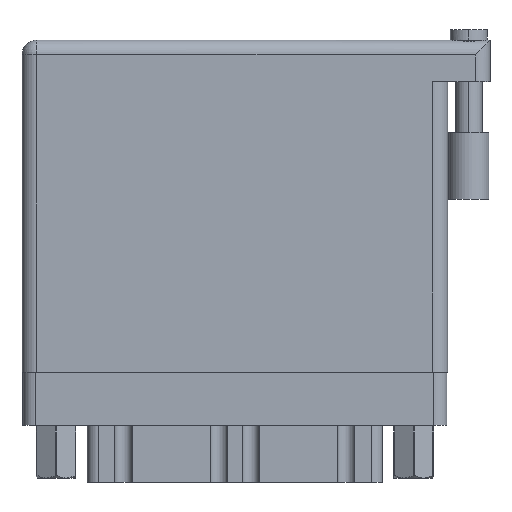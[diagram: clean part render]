
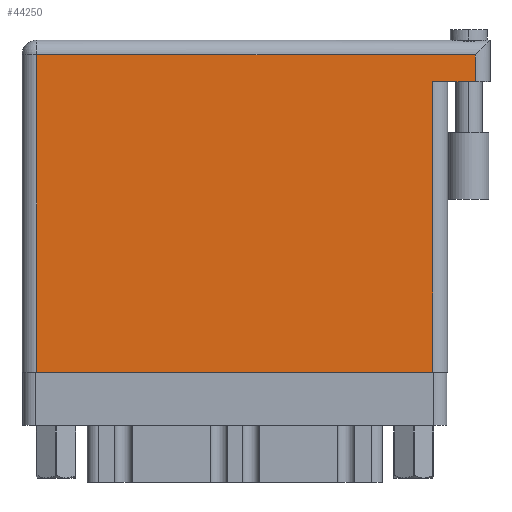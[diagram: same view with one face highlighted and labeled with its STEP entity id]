
A CAD part, front view. The second image highlights one B-rep face of the part: STEP entity #44250.
In plain terms, the highlighted face is planar.
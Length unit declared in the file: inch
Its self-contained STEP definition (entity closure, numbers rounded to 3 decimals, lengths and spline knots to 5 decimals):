
#753 = LINE ( 'NONE', #29842, #9452 ) ;
#2338 = VERTEX_POINT ( 'NONE', #11814 ) ;
#2856 = DIRECTION ( 'NONE',  ( 0., 1., 0. ) ) ;
#3037 = CARTESIAN_POINT ( 'NONE',  ( 0.07, 0., 0. ) ) ;
#3648 = CARTESIAN_POINT ( 'NONE',  ( 2.138, 1.496, 0. ) ) ;
#4617 = VECTOR ( 'NONE', #2856, 39.37008 ) ;
#7962 = VECTOR ( 'NONE', #34543, 39.37008 ) ;
#8589 = CARTESIAN_POINT ( 'NONE',  ( 0.07, 0., 0. ) ) ;
#8846 = VERTEX_POINT ( 'NONE', #3648 ) ;
#9449 = CARTESIAN_POINT ( 'NONE',  ( 0., 1.566, 0. ) ) ;
#9452 = VECTOR ( 'NONE', #19588, 39.37008 ) ;
#10543 = ORIENTED_EDGE ( 'NONE', *, *, #22997, .T. ) ;
#10913 = VERTEX_POINT ( 'NONE', #41477 ) ;
#10958 = CARTESIAN_POINT ( 'NONE',  ( 2.138, 1.566, 0. ) ) ;
#11483 = CARTESIAN_POINT ( 'NONE',  ( 1.938, 0., 0. ) ) ;
#11814 = CARTESIAN_POINT ( 'NONE',  ( 1.938, 1.369, 0. ) ) ;
#13373 = VECTOR ( 'NONE', #24714, 39.37008 ) ;
#13679 = EDGE_CURVE ( 'NONE', #39308, #15111, #753, .T. ) ;
#15111 = VERTEX_POINT ( 'NONE', #11483 ) ;
#15180 = LINE ( 'NONE', #41134, #33254 ) ;
#16439 = LINE ( 'NONE', #35491, #7962 ) ;
#16831 = DIRECTION ( 'NONE',  ( 0., 0., -1. ) ) ;
#17113 = EDGE_CURVE ( 'NONE', #8846, #10913, #31848, .T. ) ;
#19588 = DIRECTION ( 'NONE',  ( 1., 0., 0. ) ) ;
#20398 = DIRECTION ( 'NONE',  ( -1., 0., 0. ) ) ;
#22274 = ORIENTED_EDGE ( 'NONE', *, *, #25576, .T. ) ;
#22997 = EDGE_CURVE ( 'NONE', #26460, #8846, #24798, .T. ) ;
#24198 = ORIENTED_EDGE ( 'NONE', *, *, #46103, .F. ) ;
#24227 = PLANE ( 'NONE',  #34693 ) ;
#24714 = DIRECTION ( 'NONE',  ( -1., 0., 0. ) ) ;
#24798 = LINE ( 'NONE', #10958, #4617 ) ;
#25576 = EDGE_CURVE ( 'NONE', #15111, #2338, #16439, .T. ) ;
#26460 = VERTEX_POINT ( 'NONE', #27039 ) ;
#27039 = CARTESIAN_POINT ( 'NONE',  ( 2.138, 1.369, 0. ) ) ;
#28531 = LINE ( 'NONE', #3037, #29749 ) ;
#29749 = VECTOR ( 'NONE', #36144, 39.37008 ) ;
#29842 = CARTESIAN_POINT ( 'NONE',  ( 0., 0., 0. ) ) ;
#30719 = ORIENTED_EDGE ( 'NONE', *, *, #17113, .T. ) ;
#31848 = LINE ( 'NONE', #46368, #13373 ) ;
#33136 = EDGE_CURVE ( 'NONE', #10913, #39308, #28531, .T. ) ;
#33254 = VECTOR ( 'NONE', #37782, 39.37008 ) ;
#34543 = DIRECTION ( 'NONE',  ( 0., 1., 0. ) ) ;
#34693 = AXIS2_PLACEMENT_3D ( 'NONE', #9449, #16831, #20398 ) ;
#35491 = CARTESIAN_POINT ( 'NONE',  ( 1.938, 1.369, 0. ) ) ;
#36144 = DIRECTION ( 'NONE',  ( 0., -1., 0. ) ) ;
#37782 = DIRECTION ( 'NONE',  ( -1., 0., 0. ) ) ;
#39308 = VERTEX_POINT ( 'NONE', #8589 ) ;
#41134 = CARTESIAN_POINT ( 'NONE',  ( 2.208, 1.369, 0. ) ) ;
#41477 = CARTESIAN_POINT ( 'NONE',  ( 0.07, 1.496, 0. ) ) ;
#41483 = ORIENTED_EDGE ( 'NONE', *, *, #13679, .T. ) ;
#42782 = FACE_OUTER_BOUND ( 'NONE', #46001, .T. ) ;
#43671 = ORIENTED_EDGE ( 'NONE', *, *, #33136, .T. ) ;
#44250 = ADVANCED_FACE ( 'NONE', ( #42782 ), #24227, .F. ) ;
#46001 = EDGE_LOOP ( 'NONE', ( #41483, #22274, #24198, #10543, #30719, #43671 ) ) ;
#46103 = EDGE_CURVE ( 'NONE', #26460, #2338, #15180, .T. ) ;
#46368 = CARTESIAN_POINT ( 'NONE',  ( 0., 1.496, 0. ) ) ;
